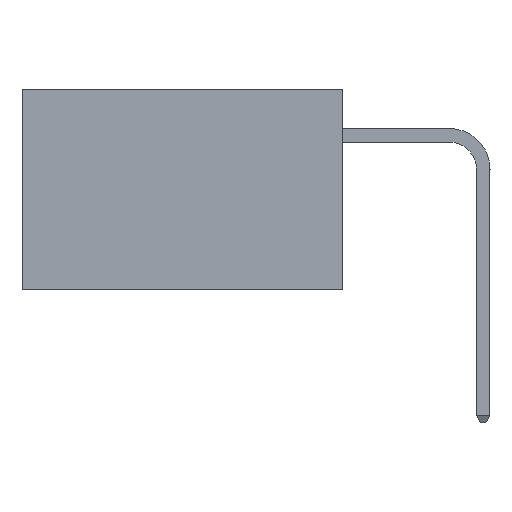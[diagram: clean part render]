
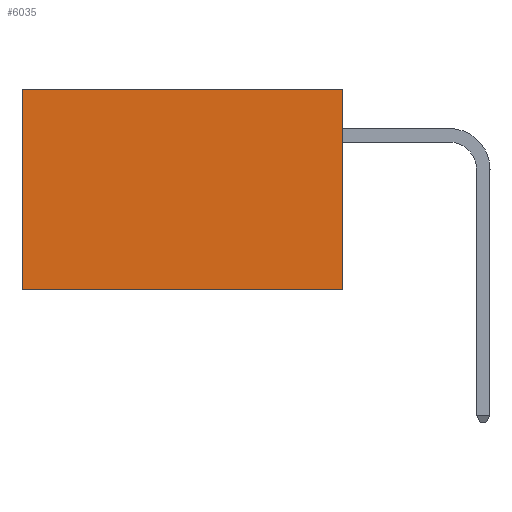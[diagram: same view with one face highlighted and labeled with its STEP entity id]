
A CAD part, left-side view. The second image highlights one B-rep face of the part: STEP entity #6035.
In plain terms, the highlighted planar face has unit normal (-1, 0, 0).
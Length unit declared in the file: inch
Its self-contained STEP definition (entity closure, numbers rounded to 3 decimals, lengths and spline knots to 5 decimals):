
#6 = VECTOR ( 'NONE', #7082, 39.37008 ) ;
#352 = VERTEX_POINT ( 'NONE', #14442 ) ;
#713 = ORIENTED_EDGE ( 'NONE', *, *, #3353, .T. ) ;
#861 = DIRECTION ( 'NONE',  ( 0., 1., 0. ) ) ;
#1195 = VERTEX_POINT ( 'NONE', #5443 ) ;
#2288 = ORIENTED_EDGE ( 'NONE', *, *, #11355, .F. ) ;
#2732 = ORIENTED_EDGE ( 'NONE', *, *, #8784, .F. ) ;
#2788 = ORIENTED_EDGE ( 'NONE', *, *, #16666, .T. ) ;
#3200 = DIRECTION ( 'NONE',  ( 0., 0., -1. ) ) ;
#3240 = DIRECTION ( 'NONE',  ( 1., 0., 0. ) ) ;
#3295 = LINE ( 'NONE', #6989, #10109 ) ;
#3338 = PLANE ( 'NONE',  #13482 ) ;
#3351 = CARTESIAN_POINT ( 'NONE',  ( 0.277, 0., -0.37 ) ) ;
#3353 = EDGE_CURVE ( 'NONE', #12301, #1195, #13305, .T. ) ;
#4584 = EDGE_LOOP ( 'NONE', ( #713, #2288, #2732, #2788 ) ) ;
#5443 = CARTESIAN_POINT ( 'NONE',  ( 0.277, 0.59, -0.37 ) ) ;
#5691 = VECTOR ( 'NONE', #861, 39.37008 ) ;
#6035 = ADVANCED_FACE ( 'NONE', ( #8878 ), #3338, .F. ) ;
#6158 = CARTESIAN_POINT ( 'NONE',  ( 0.277, 0., -0.37 ) ) ;
#6582 = VECTOR ( 'NONE', #13479, 39.37008 ) ;
#6989 = CARTESIAN_POINT ( 'NONE',  ( 0.277, 0., -0.37 ) ) ;
#7082 = DIRECTION ( 'NONE',  ( 0., 1., 0. ) ) ;
#8772 = CARTESIAN_POINT ( 'NONE',  ( 0.277, 0.59, 0. ) ) ;
#8784 = EDGE_CURVE ( 'NONE', #16185, #352, #3295, .T. ) ;
#8878 = FACE_OUTER_BOUND ( 'NONE', #4584, .T. ) ;
#10109 = VECTOR ( 'NONE', #15826, 39.37008 ) ;
#10253 = LINE ( 'NONE', #14659, #6 ) ;
#11355 = EDGE_CURVE ( 'NONE', #352, #1195, #11665, .T. ) ;
#11518 = CARTESIAN_POINT ( 'NONE',  ( 0.277, 0.59, -0.37 ) ) ;
#11665 = LINE ( 'NONE', #6158, #5691 ) ;
#12301 = VERTEX_POINT ( 'NONE', #8772 ) ;
#13305 = LINE ( 'NONE', #11518, #6582 ) ;
#13479 = DIRECTION ( 'NONE',  ( 0., 0., -1. ) ) ;
#13482 = AXIS2_PLACEMENT_3D ( 'NONE', #3351, #3240, #3200 ) ;
#14442 = CARTESIAN_POINT ( 'NONE',  ( 0.277, 0., -0.37 ) ) ;
#14659 = CARTESIAN_POINT ( 'NONE',  ( 0.277, 0., 0. ) ) ;
#15826 = DIRECTION ( 'NONE',  ( 0., 0., -1. ) ) ;
#16143 = CARTESIAN_POINT ( 'NONE',  ( 0.277, 0., 0. ) ) ;
#16185 = VERTEX_POINT ( 'NONE', #16143 ) ;
#16666 = EDGE_CURVE ( 'NONE', #16185, #12301, #10253, .T. ) ;
